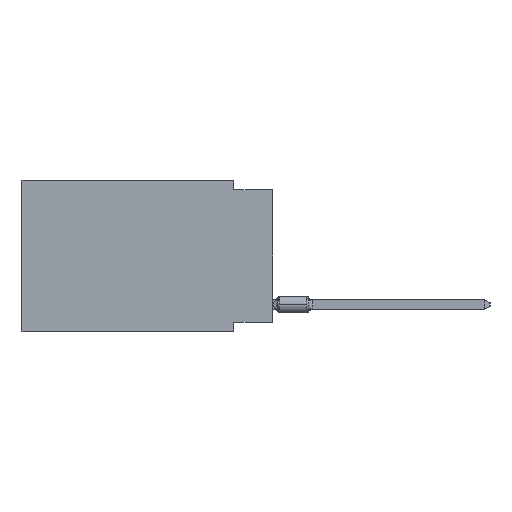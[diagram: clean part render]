
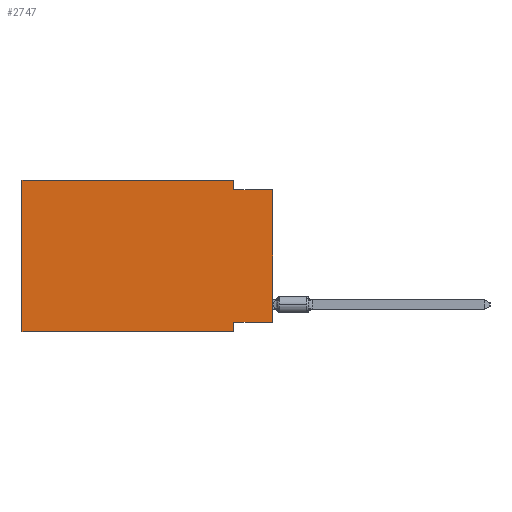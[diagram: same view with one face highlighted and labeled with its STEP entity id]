
A CAD part, left-side view. The second image highlights one B-rep face of the part: STEP entity #2747.
In plain terms, the highlighted planar face has unit normal (-1, 0, 0).
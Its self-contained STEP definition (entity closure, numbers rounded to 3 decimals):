
#404 = EDGE_CURVE ( 'NONE', #22508, #17219, #1627, .T. ) ;
#1012 = VECTOR ( 'NONE', #33462, 1000. ) ;
#1416 = CARTESIAN_POINT ( 'NONE',  ( 0., 16.383, 0. ) ) ;
#1627 = LINE ( 'NONE', #1416, #6455 ) ;
#2022 = CARTESIAN_POINT ( 'NONE',  ( 0., 0., -0.635 ) ) ;
#2055 = EDGE_CURVE ( 'NONE', #32149, #36792, #28856, .T. ) ;
#2280 = LINE ( 'NONE', #30114, #37981 ) ;
#2747 = ADVANCED_FACE ( 'NONE', ( #25462 ), #19177, .F. ) ;
#3220 = LINE ( 'NONE', #18062, #13949 ) ;
#5543 = CARTESIAN_POINT ( 'NONE',  ( 0., 16.383, 0. ) ) ;
#5880 = ORIENTED_EDGE ( 'NONE', *, *, #40203, .T. ) ;
#6455 = VECTOR ( 'NONE', #32511, 1000. ) ;
#6975 = DIRECTION ( 'NONE',  ( 0., 0., -1. ) ) ;
#8668 = LINE ( 'NONE', #21079, #1012 ) ;
#8944 = EDGE_CURVE ( 'NONE', #27601, #22508, #12241, .T. ) ;
#10219 = CARTESIAN_POINT ( 'NONE',  ( 0., 2.54, 0. ) ) ;
#11482 = CARTESIAN_POINT ( 'NONE',  ( 0., 2.54, 0. ) ) ;
#12031 = VECTOR ( 'NONE', #35585, 1000. ) ;
#12241 = LINE ( 'NONE', #5543, #12484 ) ;
#12484 = VECTOR ( 'NONE', #18535, 1000. ) ;
#12637 = VECTOR ( 'NONE', #34995, 1000. ) ;
#12880 = DIRECTION ( 'NONE',  ( 1., 0., 0. ) ) ;
#13202 = VECTOR ( 'NONE', #13794, 1000. ) ;
#13794 = DIRECTION ( 'NONE',  ( 0., 0., 1. ) ) ;
#13937 = ORIENTED_EDGE ( 'NONE', *, *, #404, .F. ) ;
#13949 = VECTOR ( 'NONE', #36552, 1000. ) ;
#14410 = EDGE_CURVE ( 'NONE', #21318, #37929, #2280, .T. ) ;
#15497 = CARTESIAN_POINT ( 'NONE',  ( 0., 16.383, -9.906 ) ) ;
#15670 = ORIENTED_EDGE ( 'NONE', *, *, #2055, .T. ) ;
#16507 = CARTESIAN_POINT ( 'NONE',  ( 0., 2.54, -9.271 ) ) ;
#17190 = CARTESIAN_POINT ( 'NONE',  ( 0., 0., -9.271 ) ) ;
#17219 = VERTEX_POINT ( 'NONE', #11482 ) ;
#17857 = EDGE_CURVE ( 'NONE', #17219, #38834, #33613, .T. ) ;
#18062 = CARTESIAN_POINT ( 'NONE',  ( 0., 0., -9.271 ) ) ;
#18535 = DIRECTION ( 'NONE',  ( 0., 0., 1. ) ) ;
#18598 = EDGE_CURVE ( 'NONE', #32149, #21318, #3220, .T. ) ;
#19177 = PLANE ( 'NONE',  #34116 ) ;
#19969 = CARTESIAN_POINT ( 'NONE',  ( 0., 16.383, 0. ) ) ;
#20508 = ORIENTED_EDGE ( 'NONE', *, *, #18598, .F. ) ;
#20773 = LINE ( 'NONE', #32527, #12031 ) ;
#21079 = CARTESIAN_POINT ( 'NONE',  ( 0., 16.383, -9.906 ) ) ;
#21318 = VERTEX_POINT ( 'NONE', #16507 ) ;
#22508 = VERTEX_POINT ( 'NONE', #19969 ) ;
#23259 = CARTESIAN_POINT ( 'NONE',  ( 0., 2.54, -0.635 ) ) ;
#23814 = CARTESIAN_POINT ( 'NONE',  ( 0., 2.54, -9.906 ) ) ;
#24666 = ORIENTED_EDGE ( 'NONE', *, *, #17857, .F. ) ;
#25462 = FACE_OUTER_BOUND ( 'NONE', #38678, .T. ) ;
#27601 = VERTEX_POINT ( 'NONE', #15497 ) ;
#28856 = LINE ( 'NONE', #38593, #13202 ) ;
#29082 = ORIENTED_EDGE ( 'NONE', *, *, #39168, .F. ) ;
#29184 = ORIENTED_EDGE ( 'NONE', *, *, #14410, .F. ) ;
#30114 = CARTESIAN_POINT ( 'NONE',  ( 0., 2.54, -9.906 ) ) ;
#31278 = ORIENTED_EDGE ( 'NONE', *, *, #8944, .F. ) ;
#32149 = VERTEX_POINT ( 'NONE', #17190 ) ;
#32511 = DIRECTION ( 'NONE',  ( 0., -1., 0. ) ) ;
#32527 = CARTESIAN_POINT ( 'NONE',  ( 0., 0., -0.635 ) ) ;
#33462 = DIRECTION ( 'NONE',  ( 0., -1., 0. ) ) ;
#33613 = LINE ( 'NONE', #10219, #12637 ) ;
#34116 = AXIS2_PLACEMENT_3D ( 'NONE', #34810, #12880, #6975 ) ;
#34810 = CARTESIAN_POINT ( 'NONE',  ( 0., 16.383, 0. ) ) ;
#34995 = DIRECTION ( 'NONE',  ( 0., 0., -1. ) ) ;
#35585 = DIRECTION ( 'NONE',  ( 0., -1., 0. ) ) ;
#35999 = DIRECTION ( 'NONE',  ( 0., 0., -1. ) ) ;
#36552 = DIRECTION ( 'NONE',  ( 0., 1., 0. ) ) ;
#36792 = VERTEX_POINT ( 'NONE', #2022 ) ;
#37929 = VERTEX_POINT ( 'NONE', #23814 ) ;
#37981 = VECTOR ( 'NONE', #35999, 1000. ) ;
#38593 = CARTESIAN_POINT ( 'NONE',  ( 0., 0., 0. ) ) ;
#38678 = EDGE_LOOP ( 'NONE', ( #15670, #29082, #24666, #13937, #31278, #5880, #29184, #20508 ) ) ;
#38834 = VERTEX_POINT ( 'NONE', #23259 ) ;
#39168 = EDGE_CURVE ( 'NONE', #38834, #36792, #20773, .T. ) ;
#40203 = EDGE_CURVE ( 'NONE', #27601, #37929, #8668, .T. ) ;
